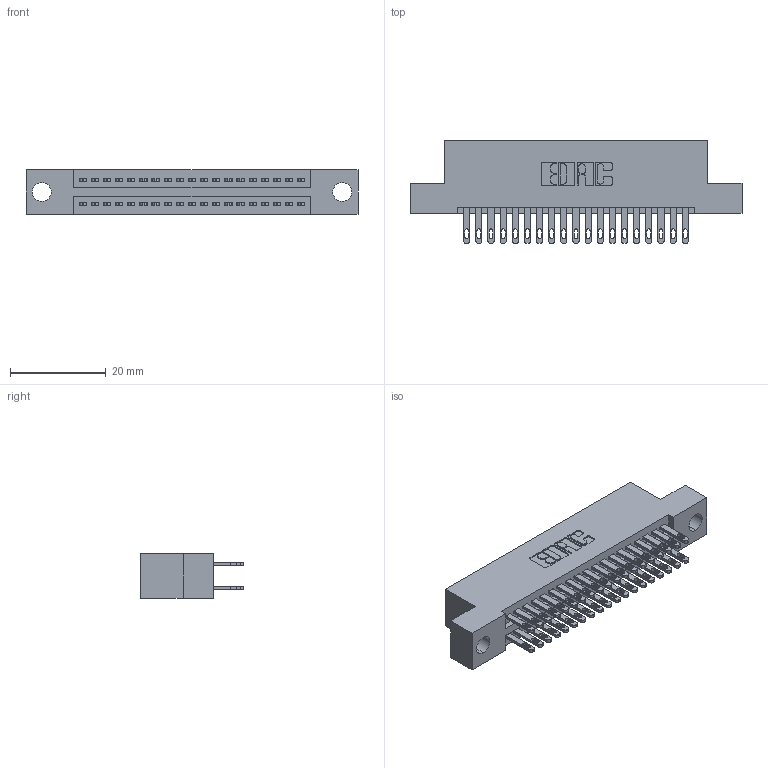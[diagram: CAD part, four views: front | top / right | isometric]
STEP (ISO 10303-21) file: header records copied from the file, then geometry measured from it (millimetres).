
FILE_DESCRIPTION (( 'STEP AP203' ), '1' );
FILE_NAME ('345-038-500-204.STEP', '2021-05-20T00:38:10', ( '' ), ( '' ), 'SwSTEP 2.0', 'SolidWorks 2020', '' );
FILE_SCHEMA (( 'CONFIG_CONTROL_DESIGN' ));
Length unit declared in the file: inch
Products named in the file (3): 345-038-500-204; 345-292-001_345-293-100; 345 Part_Flush Mounting Lugs - 0.156 Dia-TI
Assembly tree (39 placements, depth 2):
  345-038-500-204
    345 Part_Flush Mounting Lugs - 0.156 Dia-TI
    345-292-001_345-293-100  x38
Bounding box: 69.47 x 21.51 x 9.4 mm (x, y, z)
Volume: 6545 mm3; surface area: 9468.3 mm2
Topology: 39 solids, 39 shells, 1888 faces, 5735 edges, 3822 vertices
Faces by surface type: plane 1120, cylinder 768
Entity records: 18353 total; most frequent: CARTESIAN_POINT 3102, ORIENTED_EDGE 3034, DIRECTION 2765, EDGE_CURVE 1517, VECTOR 1305, LINE 1305, VERTEX_POINT 1010, AXIS2_PLACEMENT_3D 730
